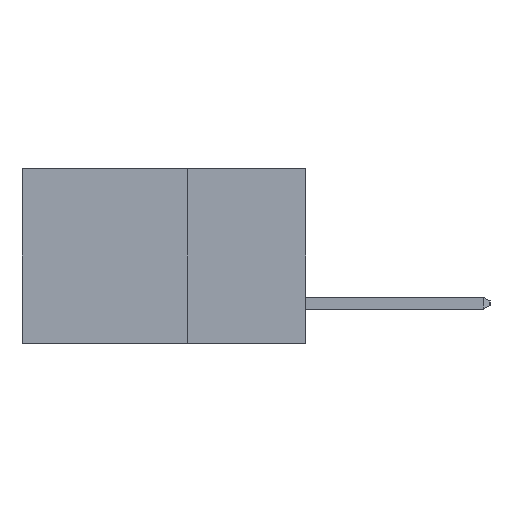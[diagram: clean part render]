
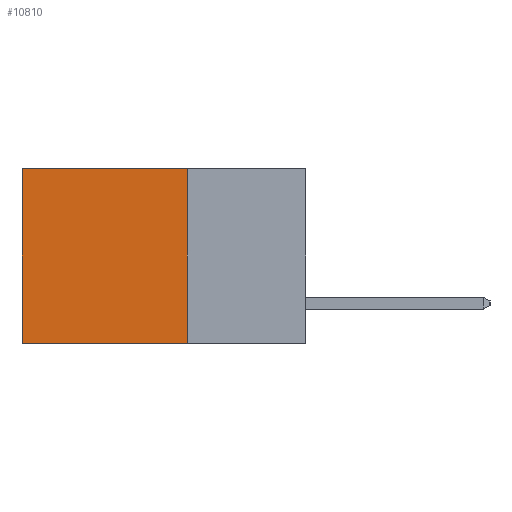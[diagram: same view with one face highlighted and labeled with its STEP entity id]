
A CAD part, left-side view. The second image highlights one B-rep face of the part: STEP entity #10810.
In plain terms, the highlighted planar face has unit normal (-1, 0, 0).
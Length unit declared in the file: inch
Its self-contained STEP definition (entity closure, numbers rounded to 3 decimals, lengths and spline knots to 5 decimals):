
#291 = VERTEX_POINT ( 'NONE', #10230 ) ;
#382 = CARTESIAN_POINT ( 'NONE',  ( 0.298, 0.25, 0. ) ) ;
#613 = VERTEX_POINT ( 'NONE', #13356 ) ;
#711 = EDGE_CURVE ( 'NONE', #4913, #17977, #8082, .T. ) ;
#1179 = DIRECTION ( 'NONE',  ( 0., 1., 0. ) ) ;
#2829 = CARTESIAN_POINT ( 'NONE',  ( 0.298, 0.25, -0.37 ) ) ;
#3275 = EDGE_CURVE ( 'NONE', #613, #291, #14663, .T. ) ;
#4913 = VERTEX_POINT ( 'NONE', #5000 ) ;
#5000 = CARTESIAN_POINT ( 'NONE',  ( 0.298, 0.25, 0. ) ) ;
#5422 = VECTOR ( 'NONE', #1179, 39.37008 ) ;
#6041 = VECTOR ( 'NONE', #11491, 39.37008 ) ;
#6418 = CARTESIAN_POINT ( 'NONE',  ( 0.298, 0.25, 0. ) ) ;
#6936 = CARTESIAN_POINT ( 'NONE',  ( 0.298, 0.6, 0. ) ) ;
#7494 = VECTOR ( 'NONE', #9692, 39.37008 ) ;
#8082 = LINE ( 'NONE', #382, #20088 ) ;
#8682 = ORIENTED_EDGE ( 'NONE', *, *, #711, .T. ) ;
#9692 = DIRECTION ( 'NONE',  ( 0., 0., -1. ) ) ;
#9961 = DIRECTION ( 'NONE',  ( 0., 1., 0. ) ) ;
#10230 = CARTESIAN_POINT ( 'NONE',  ( 0.298, 0.6, -0.37 ) ) ;
#10438 = LINE ( 'NONE', #21198, #6041 ) ;
#10810 = ADVANCED_FACE ( 'NONE', ( #19354 ), #21009, .F. ) ;
#11359 = DIRECTION ( 'NONE',  ( 0., 0., -1. ) ) ;
#11491 = DIRECTION ( 'NONE',  ( 0., 0., -1. ) ) ;
#12893 = LINE ( 'NONE', #6418, #7494 ) ;
#13356 = CARTESIAN_POINT ( 'NONE',  ( 0.298, 0.25, -0.37 ) ) ;
#13722 = EDGE_CURVE ( 'NONE', #4913, #613, #12893, .T. ) ;
#14325 = AXIS2_PLACEMENT_3D ( 'NONE', #16178, #21072, #11359 ) ;
#14663 = LINE ( 'NONE', #2829, #5422 ) ;
#15364 = ORIENTED_EDGE ( 'NONE', *, *, #13722, .F. ) ;
#16178 = CARTESIAN_POINT ( 'NONE',  ( 0.298, 0.25, 0. ) ) ;
#17357 = ORIENTED_EDGE ( 'NONE', *, *, #3275, .F. ) ;
#17977 = VERTEX_POINT ( 'NONE', #6936 ) ;
#18576 = EDGE_LOOP ( 'NONE', ( #21154, #17357, #15364, #8682 ) ) ;
#19354 = FACE_OUTER_BOUND ( 'NONE', #18576, .T. ) ;
#20088 = VECTOR ( 'NONE', #9961, 39.37008 ) ;
#20839 = EDGE_CURVE ( 'NONE', #17977, #291, #10438, .T. ) ;
#21009 = PLANE ( 'NONE',  #14325 ) ;
#21072 = DIRECTION ( 'NONE',  ( 1., 0., 0. ) ) ;
#21154 = ORIENTED_EDGE ( 'NONE', *, *, #20839, .T. ) ;
#21198 = CARTESIAN_POINT ( 'NONE',  ( 0.298, 0.6, 0. ) ) ;
